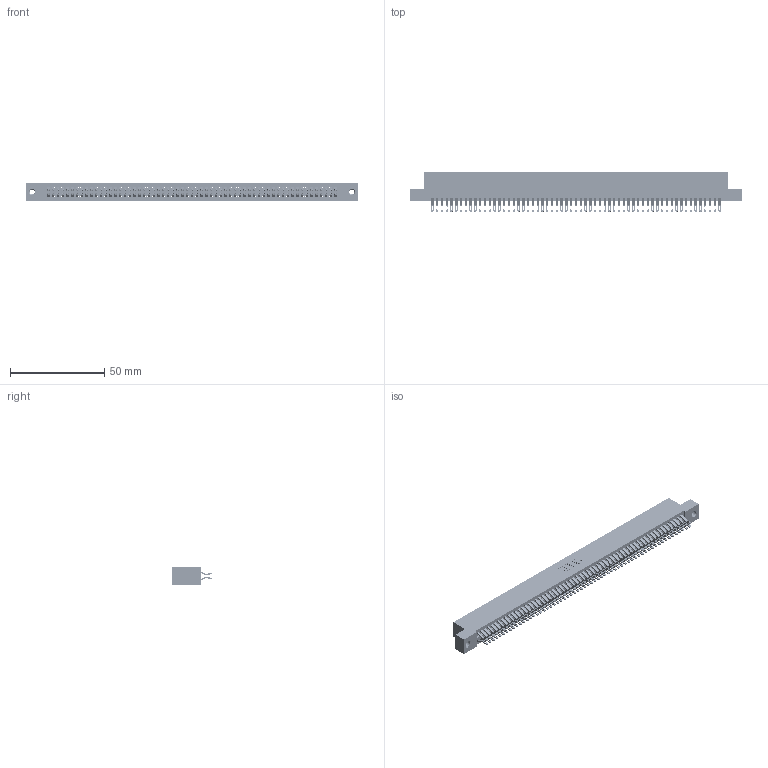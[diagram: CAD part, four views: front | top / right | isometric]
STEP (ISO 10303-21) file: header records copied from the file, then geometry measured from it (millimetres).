
FILE_DESCRIPTION (( 'STEP AP203' ), '1' );
FILE_NAME ('395-122-555-207.STEP', '2018-12-03T19:28:39', ( '' ), ( '' ), 'SwSTEP 2.0', 'SolidWorks 2016', '' );
FILE_SCHEMA (( 'CONFIG_CONTROL_DESIGN' ));
Length unit declared in the file: inch
Products named in the file (4): 395-122-555-207; 345-250-001_345-250-005-103; 345 Part_Flush Mounting Lugs - 0.156 Dia-TI; 345-292-001_555 Tail
Assembly tree (125 placements, depth 2):
  395-122-555-207
    345 Part_Flush Mounting Lugs - 0.156 Dia-TI
    345-292-001_555 Tail  x122
    345-250-001_345-250-005-103  x2
Bounding box: 176.15 x 21.13 x 9.4 mm (x, y, z)
Volume: 17628 mm3; surface area: 27683.8 mm2
Topology: 125 solids, 125 shells, 7018 faces, 22071 edges, 14706 vertices
Faces by surface type: plane 3894, cylinder 3108, cone 12, torus 4
Entity records: 46816 total; most frequent: CARTESIAN_POINT 7845, ORIENTED_EDGE 7742, DIRECTION 6889, EDGE_CURVE 3871, LINE 3455, VECTOR 3455, VERTEX_POINT 2576, AXIS2_PLACEMENT_3D 1717
